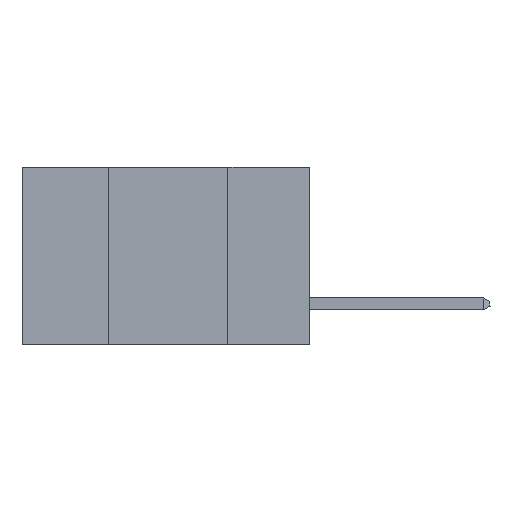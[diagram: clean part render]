
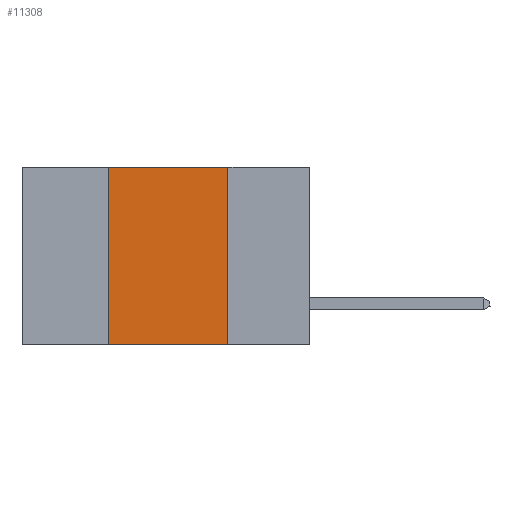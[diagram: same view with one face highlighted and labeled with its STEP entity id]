
A CAD part, left-side view. The second image highlights one B-rep face of the part: STEP entity #11308.
In plain terms, the highlighted planar face has unit normal (-1, 0, 0).
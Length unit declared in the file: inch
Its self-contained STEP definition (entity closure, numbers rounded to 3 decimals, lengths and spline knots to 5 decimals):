
#221 = VECTOR ( 'NONE', #16089, 39.37008 ) ;
#443 = VECTOR ( 'NONE', #21347, 39.37008 ) ;
#1460 = ORIENTED_EDGE ( 'NONE', *, *, #5441, .F. ) ;
#1571 = ORIENTED_EDGE ( 'NONE', *, *, #10502, .F. ) ;
#1894 = PLANE ( 'NONE',  #14340 ) ;
#2431 = CARTESIAN_POINT ( 'NONE',  ( 0., 0.17, -0.37 ) ) ;
#3673 = DIRECTION ( 'NONE',  ( 1., 0., 0. ) ) ;
#3751 = CARTESIAN_POINT ( 'NONE',  ( 0., 0.6, 0. ) ) ;
#4364 = DIRECTION ( 'NONE',  ( 0., -1., 0. ) ) ;
#5441 = EDGE_CURVE ( 'NONE', #11281, #17190, #21044, .T. ) ;
#5492 = CARTESIAN_POINT ( 'NONE',  ( 0., 0.42, 0. ) ) ;
#6774 = LINE ( 'NONE', #19553, #221 ) ;
#7022 = EDGE_LOOP ( 'NONE', ( #1571, #1460, #14150, #14590 ) ) ;
#7417 = CARTESIAN_POINT ( 'NONE',  ( 0., 0.42, 0. ) ) ;
#7793 = VERTEX_POINT ( 'NONE', #2431 ) ;
#9207 = VECTOR ( 'NONE', #21244, 39.37008 ) ;
#10477 = DIRECTION ( 'NONE',  ( 0., 0., -1. ) ) ;
#10502 = EDGE_CURVE ( 'NONE', #17190, #7793, #6774, .T. ) ;
#10533 = EDGE_CURVE ( 'NONE', #15290, #11281, #13782, .T. ) ;
#10968 = CARTESIAN_POINT ( 'NONE',  ( 0., 0.6, -0.37 ) ) ;
#11281 = VERTEX_POINT ( 'NONE', #5492 ) ;
#11308 = ADVANCED_FACE ( 'NONE', ( #20239 ), #1894, .F. ) ;
#11894 = CARTESIAN_POINT ( 'NONE',  ( 0., 0.42, -0.37 ) ) ;
#13782 = LINE ( 'NONE', #7417, #9207 ) ;
#14150 = ORIENTED_EDGE ( 'NONE', *, *, #10533, .F. ) ;
#14340 = AXIS2_PLACEMENT_3D ( 'NONE', #3751, #3673, #10477 ) ;
#14500 = CARTESIAN_POINT ( 'NONE',  ( 0., 0.17, 0. ) ) ;
#14590 = ORIENTED_EDGE ( 'NONE', *, *, #15188, .T. ) ;
#15188 = EDGE_CURVE ( 'NONE', #15290, #7793, #19395, .T. ) ;
#15290 = VERTEX_POINT ( 'NONE', #11894 ) ;
#16089 = DIRECTION ( 'NONE',  ( 0., 0., -1. ) ) ;
#16208 = CARTESIAN_POINT ( 'NONE',  ( 0., 0.6, 0. ) ) ;
#17190 = VERTEX_POINT ( 'NONE', #14500 ) ;
#19395 = LINE ( 'NONE', #10968, #443 ) ;
#19553 = CARTESIAN_POINT ( 'NONE',  ( 0., 0.17, 0. ) ) ;
#19940 = VECTOR ( 'NONE', #4364, 39.37008 ) ;
#20239 = FACE_OUTER_BOUND ( 'NONE', #7022, .T. ) ;
#21044 = LINE ( 'NONE', #16208, #19940 ) ;
#21244 = DIRECTION ( 'NONE',  ( 0., 0., 1. ) ) ;
#21347 = DIRECTION ( 'NONE',  ( 0., -1., 0. ) ) ;
